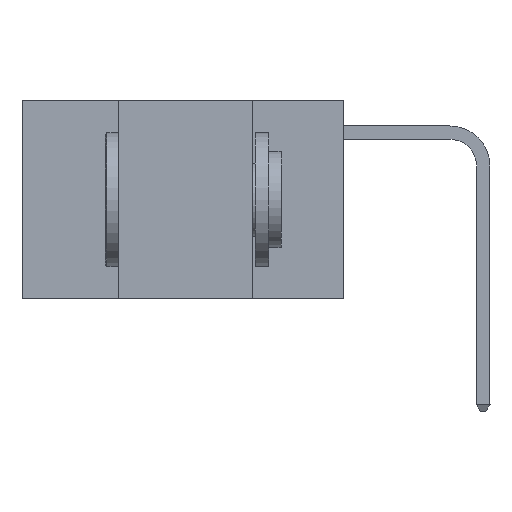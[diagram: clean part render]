
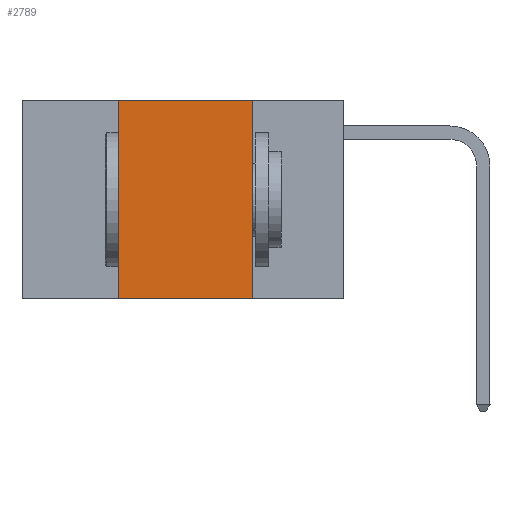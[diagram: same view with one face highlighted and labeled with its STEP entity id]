
A CAD part, left-side view. The second image highlights one B-rep face of the part: STEP entity #2789.
In plain terms, the highlighted planar face has unit normal (-1, 0, 0).
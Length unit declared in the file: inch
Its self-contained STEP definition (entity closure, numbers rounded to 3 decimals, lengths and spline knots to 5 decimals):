
#901 = CARTESIAN_POINT ( 'NONE',  ( 0., 0.17, 0. ) ) ;
#1333 = CARTESIAN_POINT ( 'NONE',  ( 0., 0.6, -0.37 ) ) ;
#1449 = CARTESIAN_POINT ( 'NONE',  ( 0., 0.42, 0. ) ) ;
#2789 = ADVANCED_FACE ( 'NONE', ( #23580 ), #26195, .F. ) ;
#3103 = EDGE_CURVE ( 'NONE', #13408, #4906, #5493, .T. ) ;
#4906 = VERTEX_POINT ( 'NONE', #1449 ) ;
#5493 = LINE ( 'NONE', #27587, #21385 ) ;
#5576 = EDGE_LOOP ( 'NONE', ( #24376, #6964, #18393, #25474 ) ) ;
#6381 = LINE ( 'NONE', #8133, #27360 ) ;
#6964 = ORIENTED_EDGE ( 'NONE', *, *, #13664, .F. ) ;
#7703 = VECTOR ( 'NONE', #26994, 39.37008 ) ;
#8133 = CARTESIAN_POINT ( 'NONE',  ( 0., 0.6, 0. ) ) ;
#8798 = LINE ( 'NONE', #1333, #16245 ) ;
#9992 = EDGE_CURVE ( 'NONE', #13408, #28634, #8798, .T. ) ;
#11667 = DIRECTION ( 'NONE',  ( 0., 0., -1. ) ) ;
#12844 = AXIS2_PLACEMENT_3D ( 'NONE', #30478, #28566, #11667 ) ;
#13408 = VERTEX_POINT ( 'NONE', #16722 ) ;
#13664 = EDGE_CURVE ( 'NONE', #4906, #24268, #6381, .T. ) ;
#15189 = DIRECTION ( 'NONE',  ( 0., 0., 1. ) ) ;
#16245 = VECTOR ( 'NONE', #22920, 39.37008 ) ;
#16722 = CARTESIAN_POINT ( 'NONE',  ( 0., 0.42, -0.37 ) ) ;
#17976 = CARTESIAN_POINT ( 'NONE',  ( 0., 0.17, 0. ) ) ;
#18393 = ORIENTED_EDGE ( 'NONE', *, *, #3103, .F. ) ;
#18436 = DIRECTION ( 'NONE',  ( 0., -1., 0. ) ) ;
#21385 = VECTOR ( 'NONE', #15189, 39.37008 ) ;
#22434 = EDGE_CURVE ( 'NONE', #24268, #28634, #24977, .T. ) ;
#22920 = DIRECTION ( 'NONE',  ( 0., -1., 0. ) ) ;
#23580 = FACE_OUTER_BOUND ( 'NONE', #5576, .T. ) ;
#23642 = CARTESIAN_POINT ( 'NONE',  ( 0., 0.17, -0.37 ) ) ;
#24268 = VERTEX_POINT ( 'NONE', #17976 ) ;
#24376 = ORIENTED_EDGE ( 'NONE', *, *, #22434, .F. ) ;
#24977 = LINE ( 'NONE', #901, #7703 ) ;
#25474 = ORIENTED_EDGE ( 'NONE', *, *, #9992, .T. ) ;
#26195 = PLANE ( 'NONE',  #12844 ) ;
#26994 = DIRECTION ( 'NONE',  ( 0., 0., -1. ) ) ;
#27360 = VECTOR ( 'NONE', #18436, 39.37008 ) ;
#27587 = CARTESIAN_POINT ( 'NONE',  ( 0., 0.42, 0. ) ) ;
#28566 = DIRECTION ( 'NONE',  ( 1., 0., 0. ) ) ;
#28634 = VERTEX_POINT ( 'NONE', #23642 ) ;
#30478 = CARTESIAN_POINT ( 'NONE',  ( 0., 0.6, 0. ) ) ;
